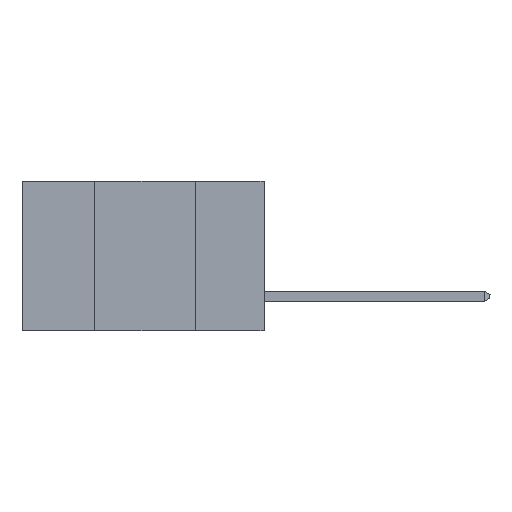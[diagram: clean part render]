
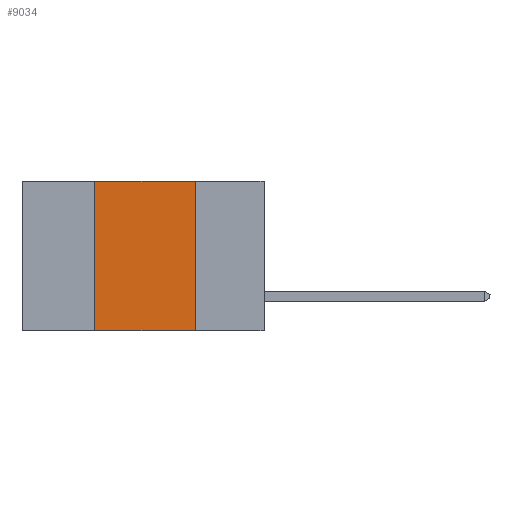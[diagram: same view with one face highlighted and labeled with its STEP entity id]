
A CAD part, left-side view. The second image highlights one B-rep face of the part: STEP entity #9034.
In plain terms, the highlighted planar face has unit normal (-1, 0, 0).
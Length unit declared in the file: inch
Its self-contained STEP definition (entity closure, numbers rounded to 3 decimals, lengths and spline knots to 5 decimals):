
#741 = DIRECTION ( 'NONE',  ( 1., 0., 0. ) ) ;
#1440 = EDGE_LOOP ( 'NONE', ( #5248, #3883, #11982, #2933 ) ) ;
#1797 = DIRECTION ( 'NONE',  ( 0., 0., -1. ) ) ;
#2933 = ORIENTED_EDGE ( 'NONE', *, *, #10690, .T. ) ;
#2946 = VECTOR ( 'NONE', #11477, 39.37008 ) ;
#3277 = CARTESIAN_POINT ( 'NONE',  ( 0., 0.6, -0.37 ) ) ;
#3883 = ORIENTED_EDGE ( 'NONE', *, *, #7276, .F. ) ;
#4374 = CARTESIAN_POINT ( 'NONE',  ( 0., 0.42, -0.37 ) ) ;
#4413 = CARTESIAN_POINT ( 'NONE',  ( 0., 0.6, 0. ) ) ;
#5248 = ORIENTED_EDGE ( 'NONE', *, *, #6370, .F. ) ;
#5567 = FACE_OUTER_BOUND ( 'NONE', #1440, .T. ) ;
#6311 = VERTEX_POINT ( 'NONE', #8842 ) ;
#6317 = LINE ( 'NONE', #6480, #2946 ) ;
#6370 = EDGE_CURVE ( 'NONE', #13637, #11176, #6317, .T. ) ;
#6480 = CARTESIAN_POINT ( 'NONE',  ( 0., 0.17, -0.37 ) ) ;
#6874 = VECTOR ( 'NONE', #15839, 39.37008 ) ;
#7065 = LINE ( 'NONE', #3277, #6874 ) ;
#7092 = DIRECTION ( 'NONE',  ( 0., 0., 1. ) ) ;
#7276 = EDGE_CURVE ( 'NONE', #6311, #13637, #15263, .T. ) ;
#8467 = LINE ( 'NONE', #4374, #9478 ) ;
#8692 = AXIS2_PLACEMENT_3D ( 'NONE', #4413, #741, #1797 ) ;
#8784 = CARTESIAN_POINT ( 'NONE',  ( 0., 0.6, 0. ) ) ;
#8785 = EDGE_CURVE ( 'NONE', #16129, #6311, #8467, .T. ) ;
#8842 = CARTESIAN_POINT ( 'NONE',  ( 0., 0.42, 0. ) ) ;
#9034 = ADVANCED_FACE ( 'NONE', ( #5567 ), #14436, .F. ) ;
#9478 = VECTOR ( 'NONE', #7092, 39.37008 ) ;
#9875 = CARTESIAN_POINT ( 'NONE',  ( 0., 0.42, -0.37 ) ) ;
#10348 = DIRECTION ( 'NONE',  ( 0., -1., 0. ) ) ;
#10690 = EDGE_CURVE ( 'NONE', #16129, #11176, #7065, .T. ) ;
#11176 = VERTEX_POINT ( 'NONE', #15985 ) ;
#11477 = DIRECTION ( 'NONE',  ( 0., 0., -1. ) ) ;
#11847 = VECTOR ( 'NONE', #10348, 39.37008 ) ;
#11982 = ORIENTED_EDGE ( 'NONE', *, *, #8785, .F. ) ;
#13637 = VERTEX_POINT ( 'NONE', #14542 ) ;
#14436 = PLANE ( 'NONE',  #8692 ) ;
#14542 = CARTESIAN_POINT ( 'NONE',  ( 0., 0.17, 0. ) ) ;
#15263 = LINE ( 'NONE', #8784, #11847 ) ;
#15839 = DIRECTION ( 'NONE',  ( 0., -1., 0. ) ) ;
#15985 = CARTESIAN_POINT ( 'NONE',  ( 0., 0.17, -0.37 ) ) ;
#16129 = VERTEX_POINT ( 'NONE', #9875 ) ;
